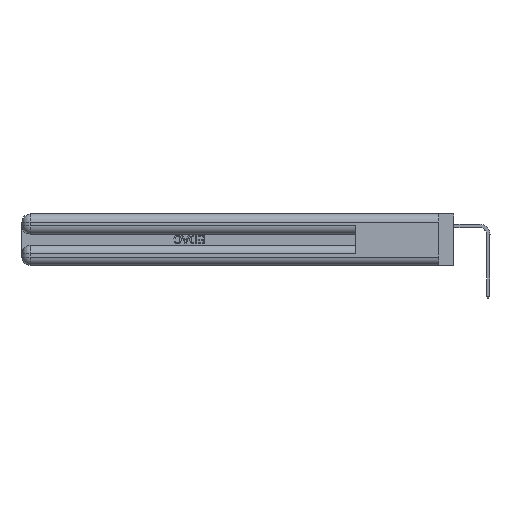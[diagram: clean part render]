
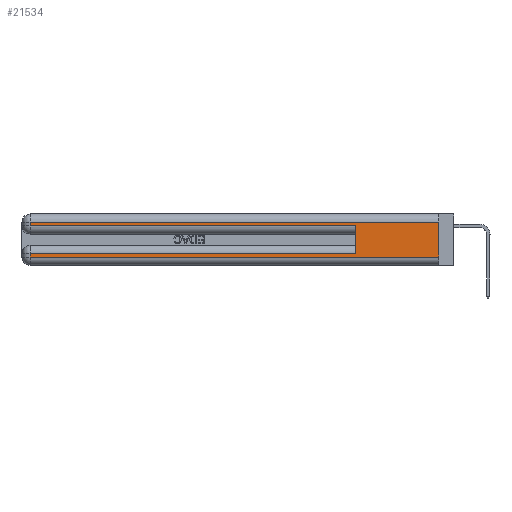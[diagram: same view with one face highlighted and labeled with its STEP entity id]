
A CAD part, left-side view. The second image highlights one B-rep face of the part: STEP entity #21534.
In plain terms, the highlighted planar face has unit normal (-1, 0, 0).
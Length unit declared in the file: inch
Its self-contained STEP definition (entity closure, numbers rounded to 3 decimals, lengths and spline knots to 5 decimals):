
#103 = VECTOR ( 'NONE', #33404, 39.37008 ) ;
#245 = EDGE_CURVE ( 'NONE', #41761, #12420, #2432, .T. ) ;
#1166 = VECTOR ( 'NONE', #20929, 39.37008 ) ;
#1491 = EDGE_CURVE ( 'NONE', #28670, #41761, #23145, .T. ) ;
#2432 = LINE ( 'NONE', #48782, #1166 ) ;
#2815 = EDGE_LOOP ( 'NONE', ( #40004, #11997, #21912, #17856, #13729, #29304, #7575, #27676 ) ) ;
#4092 = CARTESIAN_POINT ( 'NONE',  ( 0., 0.6, 0.285 ) ) ;
#4238 = DIRECTION ( 'NONE',  ( 0., 1., 0. ) ) ;
#5726 = VECTOR ( 'NONE', #22911, 39.37008 ) ;
#6413 = CARTESIAN_POINT ( 'NONE',  ( 0., 0., 0.37 ) ) ;
#7575 = ORIENTED_EDGE ( 'NONE', *, *, #11627, .T. ) ;
#8195 = VECTOR ( 'NONE', #38892, 39.37008 ) ;
#10480 = DIRECTION ( 'NONE',  ( 1., 0., 0. ) ) ;
#11627 = EDGE_CURVE ( 'NONE', #43038, #49687, #47738, .T. ) ;
#11997 = ORIENTED_EDGE ( 'NONE', *, *, #16251, .T. ) ;
#12420 = VERTEX_POINT ( 'NONE', #4092 ) ;
#12723 = DIRECTION ( 'NONE',  ( 0., 0., -1. ) ) ;
#13729 = ORIENTED_EDGE ( 'NONE', *, *, #26983, .F. ) ;
#14082 = CARTESIAN_POINT ( 'NONE',  ( 0., 0., 0.085 ) ) ;
#14087 = EDGE_CURVE ( 'NONE', #49687, #44905, #42742, .T. ) ;
#15018 = EDGE_CURVE ( 'NONE', #32783, #44905, #29570, .T. ) ;
#15259 = CARTESIAN_POINT ( 'NONE',  ( 0., 2.94, 0.37 ) ) ;
#16251 = EDGE_CURVE ( 'NONE', #32783, #28670, #46923, .T. ) ;
#17856 = ORIENTED_EDGE ( 'NONE', *, *, #245, .T. ) ;
#17868 = CARTESIAN_POINT ( 'NONE',  ( 0., 2.94, 0.06 ) ) ;
#18252 = LINE ( 'NONE', #14082, #38250 ) ;
#20034 = FACE_OUTER_BOUND ( 'NONE', #2815, .T. ) ;
#20929 = DIRECTION ( 'NONE',  ( 0., -1., 0. ) ) ;
#21534 = ADVANCED_FACE ( 'NONE', ( #20034 ), #30472, .F. ) ;
#21912 = ORIENTED_EDGE ( 'NONE', *, *, #1491, .T. ) ;
#22911 = DIRECTION ( 'NONE',  ( 0., 0., 1. ) ) ;
#23010 = CARTESIAN_POINT ( 'NONE',  ( 0., 0.6, 0.085 ) ) ;
#23145 = LINE ( 'NONE', #48667, #43092 ) ;
#26600 = DIRECTION ( 'NONE',  ( 0., 1., 0. ) ) ;
#26983 = EDGE_CURVE ( 'NONE', #38344, #12420, #38943, .T. ) ;
#27676 = ORIENTED_EDGE ( 'NONE', *, *, #14087, .T. ) ;
#27833 = VECTOR ( 'NONE', #39205, 39.37008 ) ;
#28364 = CARTESIAN_POINT ( 'NONE',  ( 0., 0., 0.31 ) ) ;
#28670 = VERTEX_POINT ( 'NONE', #42610 ) ;
#29304 = ORIENTED_EDGE ( 'NONE', *, *, #42756, .T. ) ;
#29570 = LINE ( 'NONE', #42885, #8195 ) ;
#30472 = PLANE ( 'NONE',  #42268 ) ;
#32783 = VERTEX_POINT ( 'NONE', #28364 ) ;
#33404 = DIRECTION ( 'NONE',  ( 0., -1., 0. ) ) ;
#34027 = CARTESIAN_POINT ( 'NONE',  ( 0., 2.94, 0.085 ) ) ;
#36362 = VECTOR ( 'NONE', #26600, 39.37008 ) ;
#38250 = VECTOR ( 'NONE', #4238, 39.37008 ) ;
#38344 = VERTEX_POINT ( 'NONE', #23010 ) ;
#38467 = DIRECTION ( 'NONE',  ( 0., 0., -1. ) ) ;
#38892 = DIRECTION ( 'NONE',  ( 0., 0., -1. ) ) ;
#38943 = LINE ( 'NONE', #50763, #5726 ) ;
#39205 = DIRECTION ( 'NONE',  ( 0., 0., -1. ) ) ;
#40004 = ORIENTED_EDGE ( 'NONE', *, *, #15018, .F. ) ;
#41761 = VERTEX_POINT ( 'NONE', #43012 ) ;
#42268 = AXIS2_PLACEMENT_3D ( 'NONE', #6413, #10480, #38467 ) ;
#42441 = CARTESIAN_POINT ( 'NONE',  ( 0., 0., 0.31 ) ) ;
#42610 = CARTESIAN_POINT ( 'NONE',  ( 0., 2.94, 0.31 ) ) ;
#42742 = LINE ( 'NONE', #49063, #103 ) ;
#42756 = EDGE_CURVE ( 'NONE', #38344, #43038, #18252, .T. ) ;
#42885 = CARTESIAN_POINT ( 'NONE',  ( 0., 0., 0.37 ) ) ;
#43012 = CARTESIAN_POINT ( 'NONE',  ( 0., 2.94, 0.285 ) ) ;
#43038 = VERTEX_POINT ( 'NONE', #34027 ) ;
#43092 = VECTOR ( 'NONE', #12723, 39.37008 ) ;
#44905 = VERTEX_POINT ( 'NONE', #50363 ) ;
#46923 = LINE ( 'NONE', #42441, #36362 ) ;
#47738 = LINE ( 'NONE', #15259, #27833 ) ;
#48667 = CARTESIAN_POINT ( 'NONE',  ( 0., 2.94, 0.37 ) ) ;
#48782 = CARTESIAN_POINT ( 'NONE',  ( 0., 0., 0.285 ) ) ;
#49063 = CARTESIAN_POINT ( 'NONE',  ( 0., 0., 0.06 ) ) ;
#49687 = VERTEX_POINT ( 'NONE', #17868 ) ;
#50363 = CARTESIAN_POINT ( 'NONE',  ( 0., 0., 0.06 ) ) ;
#50763 = CARTESIAN_POINT ( 'NONE',  ( 0., 0.6, 0.145 ) ) ;
